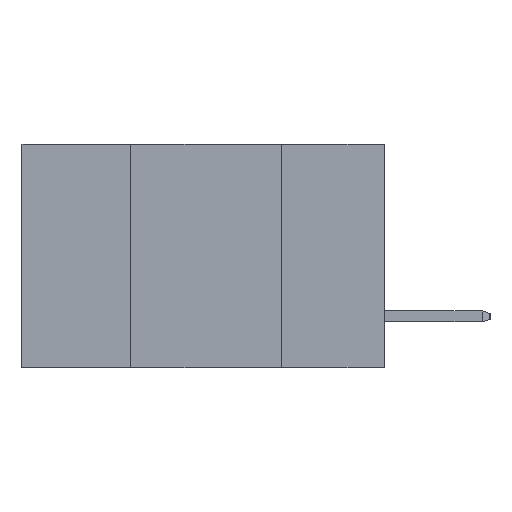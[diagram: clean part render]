
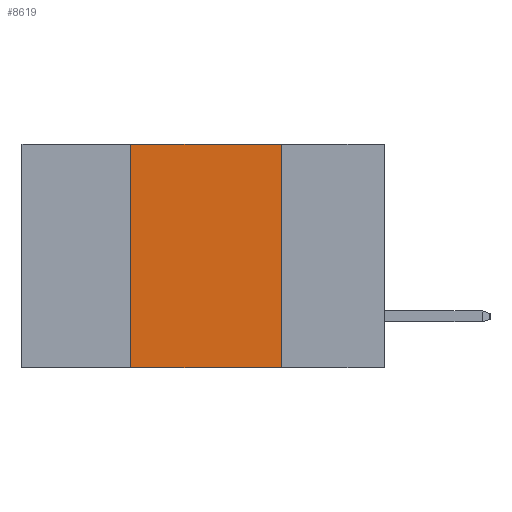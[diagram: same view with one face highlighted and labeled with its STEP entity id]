
A CAD part, left-side view. The second image highlights one B-rep face of the part: STEP entity #8619.
In plain terms, the highlighted planar face has unit normal (-1, 0, 0).
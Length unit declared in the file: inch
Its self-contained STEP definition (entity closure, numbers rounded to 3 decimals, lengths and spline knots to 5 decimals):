
#123 = EDGE_CURVE ( 'NONE', #1165, #4189, #2985, .T. ) ;
#574 = DIRECTION ( 'NONE',  ( 0., 0., 1. ) ) ;
#619 = EDGE_CURVE ( 'NONE', #1165, #8045, #8027, .T. ) ;
#684 = ORIENTED_EDGE ( 'NONE', *, *, #619, .T. ) ;
#972 = LINE ( 'NONE', #6942, #3061 ) ;
#987 = VECTOR ( 'NONE', #6040, 39.37008 ) ;
#1165 = VERTEX_POINT ( 'NONE', #7508 ) ;
#2670 = ORIENTED_EDGE ( 'NONE', *, *, #123, .F. ) ;
#2834 = CARTESIAN_POINT ( 'NONE',  ( 0., 0.42, 0. ) ) ;
#2864 = CARTESIAN_POINT ( 'NONE',  ( 0., 0.42, -0.37 ) ) ;
#2985 = LINE ( 'NONE', #2864, #6911 ) ;
#3061 = VECTOR ( 'NONE', #5559, 39.37008 ) ;
#3098 = DIRECTION ( 'NONE',  ( 1., 0., 0. ) ) ;
#3529 = DIRECTION ( 'NONE',  ( 0., 0., -1. ) ) ;
#3863 = VECTOR ( 'NONE', #3529, 39.37008 ) ;
#3880 = CARTESIAN_POINT ( 'NONE',  ( 0., 0.17, -0.37 ) ) ;
#4189 = VERTEX_POINT ( 'NONE', #2834 ) ;
#4544 = ORIENTED_EDGE ( 'NONE', *, *, #8317, .F. ) ;
#5163 = PLANE ( 'NONE',  #7763 ) ;
#5559 = DIRECTION ( 'NONE',  ( 0., -1., 0. ) ) ;
#5907 = LINE ( 'NONE', #3880, #3863 ) ;
#6022 = FACE_OUTER_BOUND ( 'NONE', #8247, .T. ) ;
#6040 = DIRECTION ( 'NONE',  ( 0., -1., 0. ) ) ;
#6173 = CARTESIAN_POINT ( 'NONE',  ( 0., 0.6, -0.37 ) ) ;
#6189 = CARTESIAN_POINT ( 'NONE',  ( 0., 0.17, 0. ) ) ;
#6911 = VECTOR ( 'NONE', #574, 39.37008 ) ;
#6942 = CARTESIAN_POINT ( 'NONE',  ( 0., 0.6, 0. ) ) ;
#7018 = EDGE_CURVE ( 'NONE', #8898, #8045, #5907, .T. ) ;
#7256 = CARTESIAN_POINT ( 'NONE',  ( 0., 0.6, 0. ) ) ;
#7266 = CARTESIAN_POINT ( 'NONE',  ( 0., 0.17, -0.37 ) ) ;
#7508 = CARTESIAN_POINT ( 'NONE',  ( 0., 0.42, -0.37 ) ) ;
#7763 = AXIS2_PLACEMENT_3D ( 'NONE', #7256, #3098, #7904 ) ;
#7904 = DIRECTION ( 'NONE',  ( 0., 0., -1. ) ) ;
#8027 = LINE ( 'NONE', #6173, #987 ) ;
#8045 = VERTEX_POINT ( 'NONE', #7266 ) ;
#8160 = ORIENTED_EDGE ( 'NONE', *, *, #7018, .F. ) ;
#8247 = EDGE_LOOP ( 'NONE', ( #8160, #4544, #2670, #684 ) ) ;
#8317 = EDGE_CURVE ( 'NONE', #4189, #8898, #972, .T. ) ;
#8619 = ADVANCED_FACE ( 'NONE', ( #6022 ), #5163, .F. ) ;
#8898 = VERTEX_POINT ( 'NONE', #6189 ) ;
